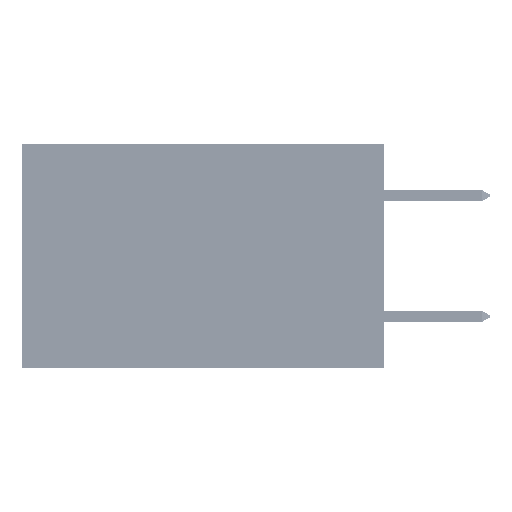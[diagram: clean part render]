
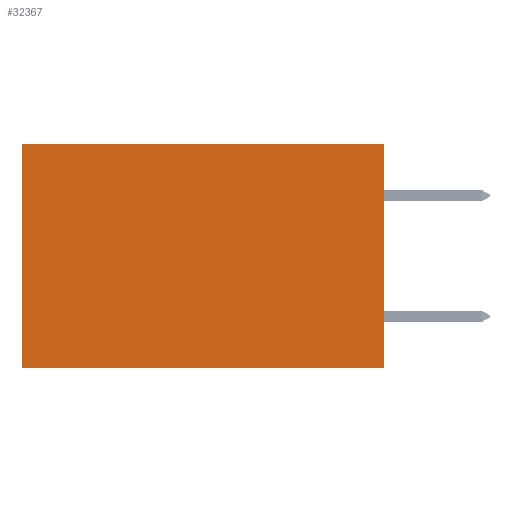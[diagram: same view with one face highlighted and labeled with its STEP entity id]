
A CAD part, left-side view. The second image highlights one B-rep face of the part: STEP entity #32367.
In plain terms, the highlighted planar face has unit normal (-1, 0, 0).
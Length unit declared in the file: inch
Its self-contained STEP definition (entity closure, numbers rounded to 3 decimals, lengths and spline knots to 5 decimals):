
#616 = CARTESIAN_POINT ( 'NONE',  ( 0.2875, 0., 0. ) ) ;
#860 = CARTESIAN_POINT ( 'NONE',  ( 0.2875, 0.6, 0. ) ) ;
#1918 = DIRECTION ( 'NONE',  ( 0., 0., -1. ) ) ;
#2036 = VERTEX_POINT ( 'NONE', #19324 ) ;
#2702 = ORIENTED_EDGE ( 'NONE', *, *, #13637, .F. ) ;
#2815 = PLANE ( 'NONE',  #36830 ) ;
#6381 = VECTOR ( 'NONE', #8253, 39.37008 ) ;
#8253 = DIRECTION ( 'NONE',  ( 0., 0., -1. ) ) ;
#11103 = CARTESIAN_POINT ( 'NONE',  ( 0.2875, 0., 0. ) ) ;
#11316 = DIRECTION ( 'NONE',  ( 0., 1., 0. ) ) ;
#13351 = LINE ( 'NONE', #860, #6381 ) ;
#13637 = EDGE_CURVE ( 'NONE', #37755, #2036, #43335, .T. ) ;
#18146 = CARTESIAN_POINT ( 'NONE',  ( 0.2875, 0., 0. ) ) ;
#18962 = VERTEX_POINT ( 'NONE', #48776 ) ;
#19324 = CARTESIAN_POINT ( 'NONE',  ( 0.2875, 0.6, -0.37 ) ) ;
#22116 = CARTESIAN_POINT ( 'NONE',  ( 0.2875, 0., -0.37 ) ) ;
#22215 = EDGE_CURVE ( 'NONE', #45097, #18962, #50066, .T. ) ;
#22739 = DIRECTION ( 'NONE',  ( 0., 0., -1. ) ) ;
#24467 = LINE ( 'NONE', #18146, #48484 ) ;
#30743 = DIRECTION ( 'NONE',  ( 0., 1., 0. ) ) ;
#30895 = CARTESIAN_POINT ( 'NONE',  ( 0.2875, 0., -0.37 ) ) ;
#30910 = EDGE_CURVE ( 'NONE', #45097, #37755, #24467, .T. ) ;
#31041 = CARTESIAN_POINT ( 'NONE',  ( 0.2875, 0., 0. ) ) ;
#31656 = ORIENTED_EDGE ( 'NONE', *, *, #30910, .F. ) ;
#32367 = ADVANCED_FACE ( 'NONE', ( #43866 ), #2815, .F. ) ;
#36830 = AXIS2_PLACEMENT_3D ( 'NONE', #11103, #46922, #22739 ) ;
#37271 = EDGE_CURVE ( 'NONE', #18962, #2036, #13351, .T. ) ;
#37755 = VERTEX_POINT ( 'NONE', #30895 ) ;
#39867 = VECTOR ( 'NONE', #11316, 39.37008 ) ;
#39908 = ORIENTED_EDGE ( 'NONE', *, *, #37271, .T. ) ;
#42055 = VECTOR ( 'NONE', #30743, 39.37008 ) ;
#43335 = LINE ( 'NONE', #22116, #42055 ) ;
#43866 = FACE_OUTER_BOUND ( 'NONE', #46779, .T. ) ;
#45097 = VERTEX_POINT ( 'NONE', #616 ) ;
#46657 = ORIENTED_EDGE ( 'NONE', *, *, #22215, .T. ) ;
#46779 = EDGE_LOOP ( 'NONE', ( #39908, #2702, #31656, #46657 ) ) ;
#46922 = DIRECTION ( 'NONE',  ( 1., 0., 0. ) ) ;
#48484 = VECTOR ( 'NONE', #1918, 39.37008 ) ;
#48776 = CARTESIAN_POINT ( 'NONE',  ( 0.2875, 0.6, 0. ) ) ;
#50066 = LINE ( 'NONE', #31041, #39867 ) ;
